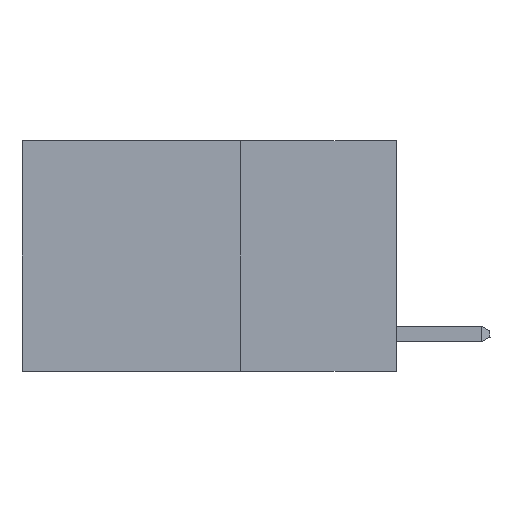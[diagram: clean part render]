
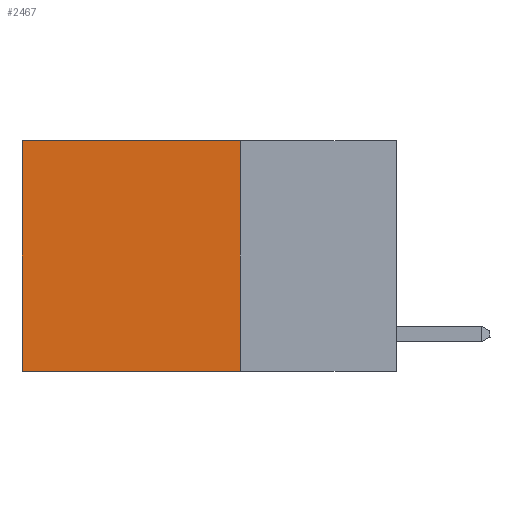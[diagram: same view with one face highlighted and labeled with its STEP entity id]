
A CAD part, left-side view. The second image highlights one B-rep face of the part: STEP entity #2467.
In plain terms, the highlighted planar face has unit normal (-1, 0, 0).
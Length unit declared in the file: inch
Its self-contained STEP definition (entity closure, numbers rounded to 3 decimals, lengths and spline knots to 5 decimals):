
#171 = ORIENTED_EDGE ( 'NONE', *, *, #19351, .T. ) ;
#846 = ORIENTED_EDGE ( 'NONE', *, *, #22074, .F. ) ;
#2003 = CARTESIAN_POINT ( 'NONE',  ( 0.2625, 0.25, 0. ) ) ;
#2467 = ADVANCED_FACE ( 'NONE', ( #15458 ), #12309, .F. ) ;
#3408 = ORIENTED_EDGE ( 'NONE', *, *, #10099, .T. ) ;
#3530 = CARTESIAN_POINT ( 'NONE',  ( 0.2625, 0.25, 0. ) ) ;
#3803 = VERTEX_POINT ( 'NONE', #17381 ) ;
#4582 = LINE ( 'NONE', #18338, #17218 ) ;
#5451 = DIRECTION ( 'NONE',  ( 0., 1., 0. ) ) ;
#6306 = LINE ( 'NONE', #13027, #11726 ) ;
#7162 = AXIS2_PLACEMENT_3D ( 'NONE', #20392, #17247, #11976 ) ;
#7345 = LINE ( 'NONE', #21123, #8875 ) ;
#8875 = VECTOR ( 'NONE', #5451, 39.37008 ) ;
#10087 = VERTEX_POINT ( 'NONE', #16659 ) ;
#10099 = EDGE_CURVE ( 'NONE', #17142, #10087, #4582, .T. ) ;
#10351 = DIRECTION ( 'NONE',  ( 0., 1., 0. ) ) ;
#11726 = VECTOR ( 'NONE', #13133, 39.37008 ) ;
#11976 = DIRECTION ( 'NONE',  ( 0., 0., -1. ) ) ;
#12082 = CARTESIAN_POINT ( 'NONE',  ( 0.2625, 0.6, 0. ) ) ;
#12309 = PLANE ( 'NONE',  #7162 ) ;
#13027 = CARTESIAN_POINT ( 'NONE',  ( 0.2625, 0.25, 0. ) ) ;
#13117 = VECTOR ( 'NONE', #10351, 39.37008 ) ;
#13133 = DIRECTION ( 'NONE',  ( 0., 0., -1. ) ) ;
#15458 = FACE_OUTER_BOUND ( 'NONE', #18470, .T. ) ;
#15823 = VERTEX_POINT ( 'NONE', #2003 ) ;
#16659 = CARTESIAN_POINT ( 'NONE',  ( 0.2625, 0.6, -0.37 ) ) ;
#17142 = VERTEX_POINT ( 'NONE', #12082 ) ;
#17218 = VECTOR ( 'NONE', #21698, 39.37008 ) ;
#17247 = DIRECTION ( 'NONE',  ( 1., 0., 0. ) ) ;
#17381 = CARTESIAN_POINT ( 'NONE',  ( 0.2625, 0.25, -0.37 ) ) ;
#18338 = CARTESIAN_POINT ( 'NONE',  ( 0.2625, 0.6, 0. ) ) ;
#18470 = EDGE_LOOP ( 'NONE', ( #3408, #20579, #846, #171 ) ) ;
#18864 = LINE ( 'NONE', #3530, #13117 ) ;
#18892 = EDGE_CURVE ( 'NONE', #3803, #10087, #7345, .T. ) ;
#19351 = EDGE_CURVE ( 'NONE', #15823, #17142, #18864, .T. ) ;
#20392 = CARTESIAN_POINT ( 'NONE',  ( 0.2625, 0.25, 0. ) ) ;
#20579 = ORIENTED_EDGE ( 'NONE', *, *, #18892, .F. ) ;
#21123 = CARTESIAN_POINT ( 'NONE',  ( 0.2625, 0.25, -0.37 ) ) ;
#21698 = DIRECTION ( 'NONE',  ( 0., 0., -1. ) ) ;
#22074 = EDGE_CURVE ( 'NONE', #15823, #3803, #6306, .T. ) ;
